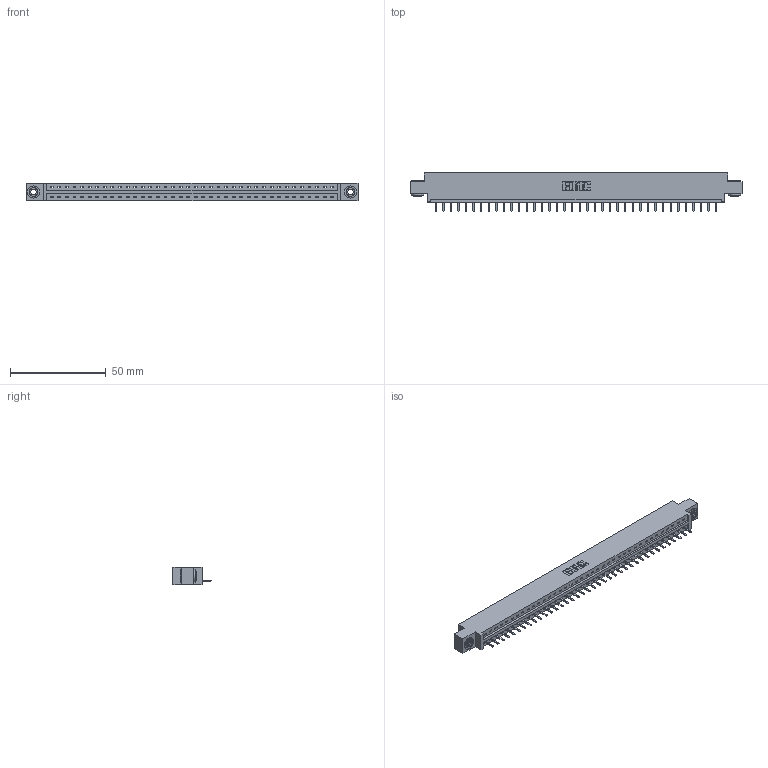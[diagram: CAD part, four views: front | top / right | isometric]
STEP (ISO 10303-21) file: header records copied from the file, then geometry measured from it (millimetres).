
FILE_DESCRIPTION (( 'STEP AP203' ), '1' );
FILE_NAME ('837-038-520-603.STEP', '2021-08-04T14:24:53', ( '' ), ( '' ), 'SwSTEP 2.0', 'SolidWorks 2020', '' );
FILE_SCHEMA (( 'CONFIG_CONTROL_DESIGN' ));
Length unit declared in the file: inch
Products named in the file (4): 345-250-002_345-250-002-102; 837 Part_0.170 Offset - 0.156 Dia-TH; 345-292-001_345-293-120; 837-038-520-603
Assembly tree (41 placements, depth 2):
  837-038-520-603
    837 Part_0.170 Offset - 0.156 Dia-TH
    345-292-001_345-293-120  x38
    345-250-002_345-250-002-102  x2
Bounding box: 173.58 x 20.02 x 9.4 mm (x, y, z)
Volume: 17783.6 mm3; surface area: 18290.2 mm2
Topology: 41 solids, 41 shells, 2664 faces, 7847 edges, 5126 vertices
Faces by surface type: plane 1908, cylinder 748, cone 8
Entity records: 29660 total; most frequent: CARTESIAN_POINT 5155, ORIENTED_EDGE 5110, DIRECTION 4369, EDGE_CURVE 2555, LINE 2399, VECTOR 2399, VERTEX_POINT 1698, AXIS2_PLACEMENT_3D 985
